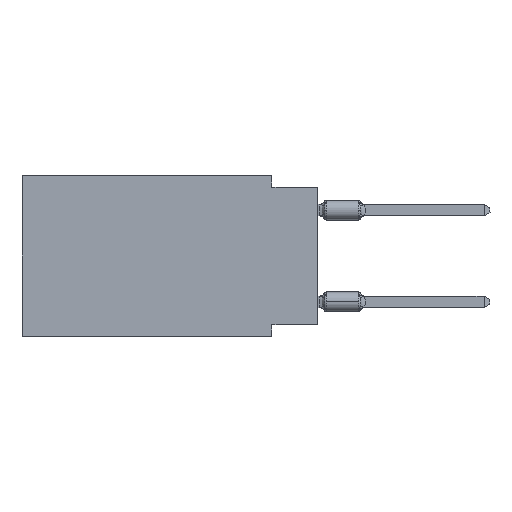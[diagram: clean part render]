
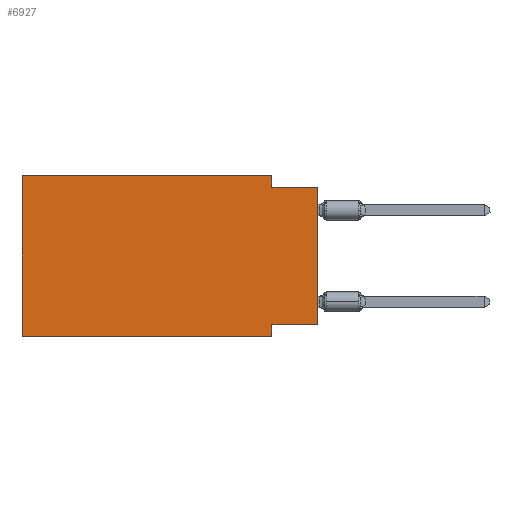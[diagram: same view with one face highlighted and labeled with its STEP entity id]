
A CAD part, left-side view. The second image highlights one B-rep face of the part: STEP entity #6927.
In plain terms, the highlighted planar face has unit normal (-1, 0, 0).
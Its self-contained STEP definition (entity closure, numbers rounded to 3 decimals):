
#468 = DIRECTION ( 'NONE',  ( 0., 1., 0. ) ) ;
#611 = PLANE ( 'NONE',  #9587 ) ;
#1064 = DIRECTION ( 'NONE',  ( 1., 0., 0. ) ) ;
#1174 = LINE ( 'NONE', #17220, #15515 ) ;
#2407 = ORIENTED_EDGE ( 'NONE', *, *, #12388, .T. ) ;
#2612 = EDGE_LOOP ( 'NONE', ( #2407, #12488, #4050, #21224, #4077, #17991, #26590, #19742 ) ) ;
#2923 = FACE_OUTER_BOUND ( 'NONE', #2612, .T. ) ;
#3185 = DIRECTION ( 'NONE',  ( 0., 0., -1. ) ) ;
#4050 = ORIENTED_EDGE ( 'NONE', *, *, #7425, .F. ) ;
#4077 = ORIENTED_EDGE ( 'NONE', *, *, #29373, .F. ) ;
#4088 = DIRECTION ( 'NONE',  ( 0., 0., -1. ) ) ;
#4640 = EDGE_CURVE ( 'NONE', #14967, #10954, #11655, .T. ) ;
#5590 = VERTEX_POINT ( 'NONE', #27127 ) ;
#5638 = LINE ( 'NONE', #9812, #18581 ) ;
#5675 = CARTESIAN_POINT ( 'NONE',  ( 0., 16.383, 0. ) ) ;
#6927 = ADVANCED_FACE ( 'NONE', ( #2923 ), #611, .F. ) ;
#7340 = CARTESIAN_POINT ( 'NONE',  ( 0., 16.383, 0. ) ) ;
#7361 = EDGE_CURVE ( 'NONE', #29915, #29138, #1174, .T. ) ;
#7425 = EDGE_CURVE ( 'NONE', #10954, #30119, #29116, .T. ) ;
#7639 = CARTESIAN_POINT ( 'NONE',  ( 0., 2.54, -8.255 ) ) ;
#8300 = VECTOR ( 'NONE', #20879, 1000. ) ;
#8841 = LINE ( 'NONE', #15496, #8300 ) ;
#9362 = DIRECTION ( 'NONE',  ( 0., 0., 1. ) ) ;
#9587 = AXIS2_PLACEMENT_3D ( 'NONE', #5675, #1064, #15084 ) ;
#9812 = CARTESIAN_POINT ( 'NONE',  ( 0., 16.383, 0. ) ) ;
#10098 = VECTOR ( 'NONE', #4088, 1000. ) ;
#10759 = EDGE_CURVE ( 'NONE', #25383, #29915, #18812, .T. ) ;
#10954 = VERTEX_POINT ( 'NONE', #24505 ) ;
#11588 = CARTESIAN_POINT ( 'NONE',  ( 0., 2.54, -8.89 ) ) ;
#11655 = LINE ( 'NONE', #7340, #29216 ) ;
#12179 = CARTESIAN_POINT ( 'NONE',  ( 0., 0., -8.255 ) ) ;
#12388 = EDGE_CURVE ( 'NONE', #25383, #20340, #16779, .T. ) ;
#12488 = ORIENTED_EDGE ( 'NONE', *, *, #24406, .F. ) ;
#13294 = DIRECTION ( 'NONE',  ( 0., -1., 0. ) ) ;
#13470 = CARTESIAN_POINT ( 'NONE',  ( 0., 2.54, -0.635 ) ) ;
#14967 = VERTEX_POINT ( 'NONE', #25537 ) ;
#15084 = DIRECTION ( 'NONE',  ( 0., 0., -1. ) ) ;
#15496 = CARTESIAN_POINT ( 'NONE',  ( 0., 16.383, -8.89 ) ) ;
#15515 = VECTOR ( 'NONE', #3185, 1000. ) ;
#16451 = CARTESIAN_POINT ( 'NONE',  ( 0., 0., -8.255 ) ) ;
#16779 = LINE ( 'NONE', #28200, #22177 ) ;
#17220 = CARTESIAN_POINT ( 'NONE',  ( 0., 2.54, -8.89 ) ) ;
#17991 = ORIENTED_EDGE ( 'NONE', *, *, #22779, .T. ) ;
#18077 = CARTESIAN_POINT ( 'NONE',  ( 0., 0., -0.635 ) ) ;
#18581 = VECTOR ( 'NONE', #28669, 1000. ) ;
#18812 = LINE ( 'NONE', #12179, #26076 ) ;
#19742 = ORIENTED_EDGE ( 'NONE', *, *, #10759, .F. ) ;
#20340 = VERTEX_POINT ( 'NONE', #20960 ) ;
#20879 = DIRECTION ( 'NONE',  ( 0., -1., 0. ) ) ;
#20960 = CARTESIAN_POINT ( 'NONE',  ( 0., 0., -0.635 ) ) ;
#21224 = ORIENTED_EDGE ( 'NONE', *, *, #4640, .F. ) ;
#21387 = DIRECTION ( 'NONE',  ( 0., -1., 0. ) ) ;
#22177 = VECTOR ( 'NONE', #9362, 1000. ) ;
#22779 = EDGE_CURVE ( 'NONE', #5590, #29138, #8841, .T. ) ;
#24406 = EDGE_CURVE ( 'NONE', #30119, #20340, #25020, .T. ) ;
#24505 = CARTESIAN_POINT ( 'NONE',  ( 0., 2.54, 0. ) ) ;
#25020 = LINE ( 'NONE', #18077, #26135 ) ;
#25383 = VERTEX_POINT ( 'NONE', #16451 ) ;
#25537 = CARTESIAN_POINT ( 'NONE',  ( 0., 16.383, 0. ) ) ;
#26076 = VECTOR ( 'NONE', #468, 1000. ) ;
#26135 = VECTOR ( 'NONE', #13294, 1000. ) ;
#26590 = ORIENTED_EDGE ( 'NONE', *, *, #7361, .F. ) ;
#27127 = CARTESIAN_POINT ( 'NONE',  ( 0., 16.383, -8.89 ) ) ;
#28200 = CARTESIAN_POINT ( 'NONE',  ( 0., 0., 0. ) ) ;
#28669 = DIRECTION ( 'NONE',  ( 0., 0., 1. ) ) ;
#29116 = LINE ( 'NONE', #29409, #10098 ) ;
#29138 = VERTEX_POINT ( 'NONE', #11588 ) ;
#29216 = VECTOR ( 'NONE', #21387, 1000. ) ;
#29373 = EDGE_CURVE ( 'NONE', #5590, #14967, #5638, .T. ) ;
#29409 = CARTESIAN_POINT ( 'NONE',  ( 0., 2.54, 0. ) ) ;
#29915 = VERTEX_POINT ( 'NONE', #7639 ) ;
#30119 = VERTEX_POINT ( 'NONE', #13470 ) ;
